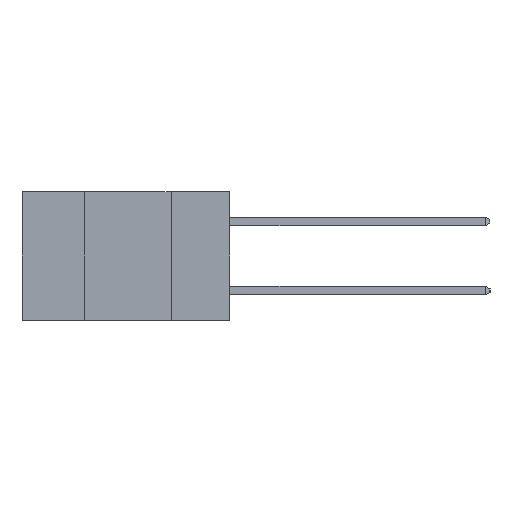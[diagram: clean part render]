
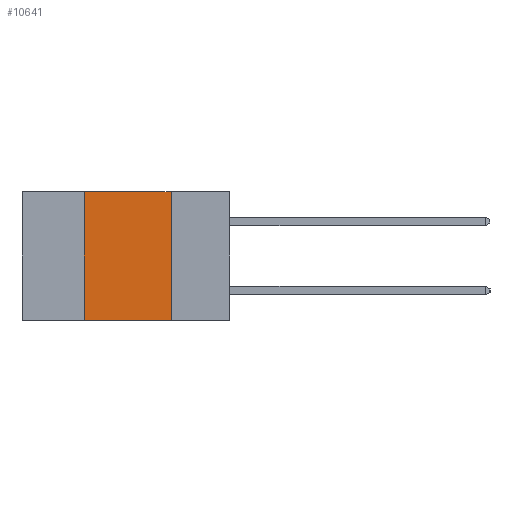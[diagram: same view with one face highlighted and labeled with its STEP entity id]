
A CAD part, left-side view. The second image highlights one B-rep face of the part: STEP entity #10641.
In plain terms, the highlighted planar face has unit normal (-1, 0, 0).
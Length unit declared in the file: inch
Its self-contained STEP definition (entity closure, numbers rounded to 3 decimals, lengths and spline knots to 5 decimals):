
#13 = ORIENTED_EDGE ( 'NONE', *, *, #446, .T. ) ;
#193 = CARTESIAN_POINT ( 'NONE',  ( 0., 0.17, -0.37 ) ) ;
#446 = EDGE_CURVE ( 'NONE', #6479, #11728, #7104, .T. ) ;
#462 = CARTESIAN_POINT ( 'NONE',  ( 0., 0.42, -0.37 ) ) ;
#616 = CARTESIAN_POINT ( 'NONE',  ( 0., 0.6, 0. ) ) ;
#771 = VECTOR ( 'NONE', #4439, 39.37008 ) ;
#890 = DIRECTION ( 'NONE',  ( 0., -1., 0. ) ) ;
#1624 = DIRECTION ( 'NONE',  ( 0., 0., -1. ) ) ;
#2322 = ORIENTED_EDGE ( 'NONE', *, *, #3556, .F. ) ;
#2555 = EDGE_LOOP ( 'NONE', ( #2322, #3088, #12640, #13 ) ) ;
#3080 = AXIS2_PLACEMENT_3D ( 'NONE', #616, #7498, #1624 ) ;
#3088 = ORIENTED_EDGE ( 'NONE', *, *, #9663, .F. ) ;
#3491 = VERTEX_POINT ( 'NONE', #7346 ) ;
#3556 = EDGE_CURVE ( 'NONE', #3491, #11728, #10894, .T. ) ;
#4405 = DIRECTION ( 'NONE',  ( 0., 0., -1. ) ) ;
#4439 = DIRECTION ( 'NONE',  ( 0., 0., 1. ) ) ;
#4511 = VECTOR ( 'NONE', #8368, 39.37008 ) ;
#5442 = LINE ( 'NONE', #10674, #10407 ) ;
#5523 = PLANE ( 'NONE',  #3080 ) ;
#5630 = VECTOR ( 'NONE', #4405, 39.37008 ) ;
#6479 = VERTEX_POINT ( 'NONE', #462 ) ;
#6592 = VERTEX_POINT ( 'NONE', #9037 ) ;
#7104 = LINE ( 'NONE', #8857, #4511 ) ;
#7346 = CARTESIAN_POINT ( 'NONE',  ( 0., 0.17, 0. ) ) ;
#7498 = DIRECTION ( 'NONE',  ( 1., 0., 0. ) ) ;
#8331 = CARTESIAN_POINT ( 'NONE',  ( 0., 0.42, -0.37 ) ) ;
#8368 = DIRECTION ( 'NONE',  ( 0., -1., 0. ) ) ;
#8857 = CARTESIAN_POINT ( 'NONE',  ( 0., 0.6, -0.37 ) ) ;
#9037 = CARTESIAN_POINT ( 'NONE',  ( 0., 0.42, 0. ) ) ;
#9417 = CARTESIAN_POINT ( 'NONE',  ( 0., 0.17, -0.37 ) ) ;
#9663 = EDGE_CURVE ( 'NONE', #6592, #3491, #5442, .T. ) ;
#10056 = FACE_OUTER_BOUND ( 'NONE', #2555, .T. ) ;
#10407 = VECTOR ( 'NONE', #890, 39.37008 ) ;
#10641 = ADVANCED_FACE ( 'NONE', ( #10056 ), #5523, .F. ) ;
#10674 = CARTESIAN_POINT ( 'NONE',  ( 0., 0.6, 0. ) ) ;
#10894 = LINE ( 'NONE', #9417, #5630 ) ;
#11265 = LINE ( 'NONE', #8331, #771 ) ;
#11728 = VERTEX_POINT ( 'NONE', #193 ) ;
#11899 = EDGE_CURVE ( 'NONE', #6479, #6592, #11265, .T. ) ;
#12640 = ORIENTED_EDGE ( 'NONE', *, *, #11899, .F. ) ;
